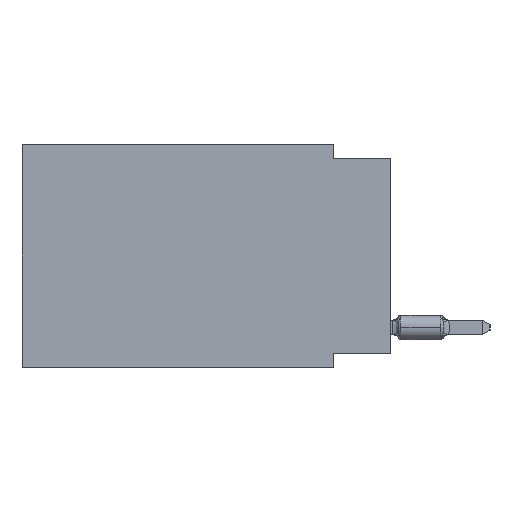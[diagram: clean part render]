
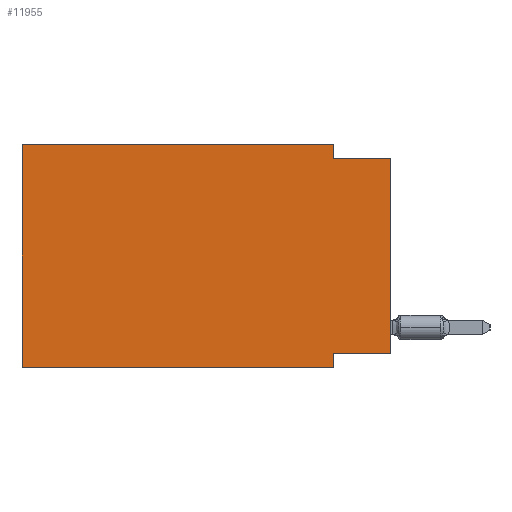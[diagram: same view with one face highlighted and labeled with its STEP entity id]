
A CAD part, left-side view. The second image highlights one B-rep face of the part: STEP entity #11955.
In plain terms, the highlighted planar face has unit normal (-1, 0, 0).
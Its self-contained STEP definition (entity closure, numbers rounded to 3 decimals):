
#2071 = DIRECTION ( 'NONE',  ( 0., 0., -1. ) ) ;
#2421 = PLANE ( 'NONE',  #29065 ) ;
#3153 = CARTESIAN_POINT ( 'NONE',  ( 0., 16.383, 0. ) ) ;
#3318 = DIRECTION ( 'NONE',  ( 0., 0., 1. ) ) ;
#5379 = EDGE_CURVE ( 'NONE', #65491, #53231, #52446, .T. ) ;
#11201 = EDGE_CURVE ( 'NONE', #41492, #25750, #58429, .T. ) ;
#11955 = ADVANCED_FACE ( 'NONE', ( #64511 ), #2421, .F. ) ;
#13705 = VECTOR ( 'NONE', #71540, 1000. ) ;
#14776 = VECTOR ( 'NONE', #52076, 1000. ) ;
#17187 = CARTESIAN_POINT ( 'NONE',  ( 0., 16.383, -9.906 ) ) ;
#17257 = EDGE_CURVE ( 'NONE', #53231, #34606, #24558, .T. ) ;
#17307 = LINE ( 'NONE', #62403, #31143 ) ;
#18658 = CARTESIAN_POINT ( 'NONE',  ( 0., 2.54, 0. ) ) ;
#19287 = CARTESIAN_POINT ( 'NONE',  ( 0., 16.383, -9.906 ) ) ;
#19612 = CARTESIAN_POINT ( 'NONE',  ( 0., 0., -9.271 ) ) ;
#19699 = ORIENTED_EDGE ( 'NONE', *, *, #5379, .F. ) ;
#21164 = CARTESIAN_POINT ( 'NONE',  ( 0., 0., -0.635 ) ) ;
#21346 = CARTESIAN_POINT ( 'NONE',  ( 0., 0., -0.635 ) ) ;
#22375 = ORIENTED_EDGE ( 'NONE', *, *, #17257, .F. ) ;
#23854 = VERTEX_POINT ( 'NONE', #39475 ) ;
#23887 = VECTOR ( 'NONE', #54919, 1000. ) ;
#24305 = EDGE_CURVE ( 'NONE', #41492, #23854, #69196, .T. ) ;
#24558 = LINE ( 'NONE', #18658, #56541 ) ;
#24808 = EDGE_CURVE ( 'NONE', #34606, #25750, #32464, .T. ) ;
#25750 = VERTEX_POINT ( 'NONE', #21164 ) ;
#25882 = CARTESIAN_POINT ( 'NONE',  ( 0., 2.54, -0.635 ) ) ;
#26301 = CARTESIAN_POINT ( 'NONE',  ( 0., 2.54, 0. ) ) ;
#26811 = LINE ( 'NONE', #60830, #13705 ) ;
#27240 = VERTEX_POINT ( 'NONE', #19287 ) ;
#27529 = LINE ( 'NONE', #17187, #23887 ) ;
#28013 = VECTOR ( 'NONE', #3318, 1000. ) ;
#28735 = DIRECTION ( 'NONE',  ( 0., 0., 1. ) ) ;
#29065 = AXIS2_PLACEMENT_3D ( 'NONE', #3153, #57887, #2071 ) ;
#31143 = VECTOR ( 'NONE', #28735, 1000. ) ;
#32464 = LINE ( 'NONE', #21346, #63712 ) ;
#34458 = DIRECTION ( 'NONE',  ( 0., 1., 0. ) ) ;
#34606 = VERTEX_POINT ( 'NONE', #25882 ) ;
#37520 = ORIENTED_EDGE ( 'NONE', *, *, #24808, .F. ) ;
#38274 = EDGE_CURVE ( 'NONE', #27240, #45395, #27529, .T. ) ;
#39475 = CARTESIAN_POINT ( 'NONE',  ( 0., 2.54, -9.271 ) ) ;
#40014 = CARTESIAN_POINT ( 'NONE',  ( 0., 0., -9.271 ) ) ;
#40536 = ORIENTED_EDGE ( 'NONE', *, *, #24305, .F. ) ;
#41492 = VERTEX_POINT ( 'NONE', #19612 ) ;
#45395 = VERTEX_POINT ( 'NONE', #59412 ) ;
#47125 = DIRECTION ( 'NONE',  ( 0., 0., -1. ) ) ;
#48165 = EDGE_CURVE ( 'NONE', #27240, #65491, #17307, .T. ) ;
#52076 = DIRECTION ( 'NONE',  ( 0., -1., 0. ) ) ;
#52446 = LINE ( 'NONE', #69071, #14776 ) ;
#53199 = EDGE_LOOP ( 'NONE', ( #70751, #37520, #22375, #19699, #63300, #55397, #62178, #40536 ) ) ;
#53231 = VERTEX_POINT ( 'NONE', #26301 ) ;
#53965 = CARTESIAN_POINT ( 'NONE',  ( 0., 0., 0. ) ) ;
#54919 = DIRECTION ( 'NONE',  ( 0., -1., 0. ) ) ;
#55379 = DIRECTION ( 'NONE',  ( 0., -1., 0. ) ) ;
#55397 = ORIENTED_EDGE ( 'NONE', *, *, #38274, .T. ) ;
#56541 = VECTOR ( 'NONE', #47125, 1000. ) ;
#57887 = DIRECTION ( 'NONE',  ( 1., 0., 0. ) ) ;
#58429 = LINE ( 'NONE', #53965, #28013 ) ;
#59412 = CARTESIAN_POINT ( 'NONE',  ( 0., 2.54, -9.906 ) ) ;
#60830 = CARTESIAN_POINT ( 'NONE',  ( 0., 2.54, -9.906 ) ) ;
#61217 = VECTOR ( 'NONE', #34458, 1000. ) ;
#62178 = ORIENTED_EDGE ( 'NONE', *, *, #69607, .F. ) ;
#62403 = CARTESIAN_POINT ( 'NONE',  ( 0., 16.383, 0. ) ) ;
#63300 = ORIENTED_EDGE ( 'NONE', *, *, #48165, .F. ) ;
#63712 = VECTOR ( 'NONE', #55379, 1000. ) ;
#64511 = FACE_OUTER_BOUND ( 'NONE', #53199, .T. ) ;
#65491 = VERTEX_POINT ( 'NONE', #67668 ) ;
#67668 = CARTESIAN_POINT ( 'NONE',  ( 0., 16.383, 0. ) ) ;
#69071 = CARTESIAN_POINT ( 'NONE',  ( 0., 16.383, 0. ) ) ;
#69196 = LINE ( 'NONE', #40014, #61217 ) ;
#69607 = EDGE_CURVE ( 'NONE', #23854, #45395, #26811, .T. ) ;
#70751 = ORIENTED_EDGE ( 'NONE', *, *, #11201, .T. ) ;
#71540 = DIRECTION ( 'NONE',  ( 0., 0., -1. ) ) ;
